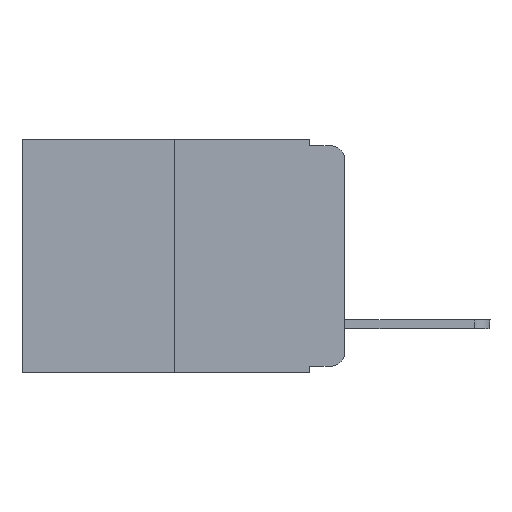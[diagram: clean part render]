
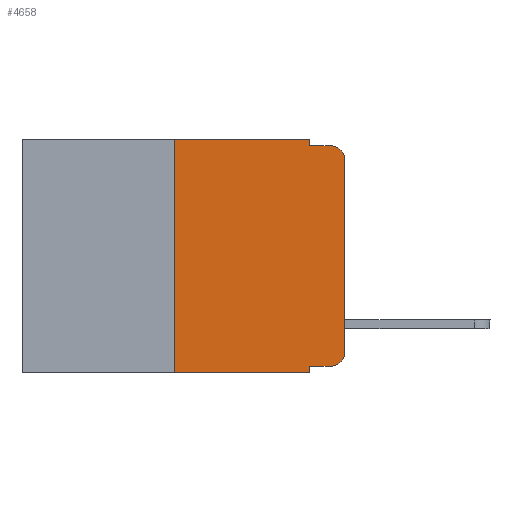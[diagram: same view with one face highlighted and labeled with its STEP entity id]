
A CAD part, left-side view. The second image highlights one B-rep face of the part: STEP entity #4658.
In plain terms, the highlighted planar face has unit normal (-1, 0, 0).
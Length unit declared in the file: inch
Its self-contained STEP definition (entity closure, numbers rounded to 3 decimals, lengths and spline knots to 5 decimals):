
#89 = VERTEX_POINT ( 'NONE', #10293 ) ;
#838 = PLANE ( 'NONE',  #9090 ) ;
#1021 = LINE ( 'NONE', #12332, #5460 ) ;
#1070 = DIRECTION ( 'NONE',  ( 0., 0., 1. ) ) ;
#1566 = VERTEX_POINT ( 'NONE', #2214 ) ;
#1743 = ORIENTED_EDGE ( 'NONE', *, *, #5074, .F. ) ;
#1755 = CARTESIAN_POINT ( 'NONE',  ( 0., 0.02, -0.333 ) ) ;
#2003 = AXIS2_PLACEMENT_3D ( 'NONE', #7945, #13956, #18308 ) ;
#2105 = VERTEX_POINT ( 'NONE', #3753 ) ;
#2194 = CIRCLE ( 'NONE', #2003, 0.02 ) ;
#2214 = CARTESIAN_POINT ( 'NONE',  ( 0., 0.051, -0.01 ) ) ;
#2468 = VECTOR ( 'NONE', #13361, 39.37008 ) ;
#2603 = EDGE_CURVE ( 'NONE', #1566, #3962, #10765, .T. ) ;
#2634 = EDGE_CURVE ( 'NONE', #2105, #3428, #10291, .T. ) ;
#3071 = CIRCLE ( 'NONE', #10545, 0.02 ) ;
#3290 = EDGE_CURVE ( 'NONE', #9376, #14216, #14406, .T. ) ;
#3428 = VERTEX_POINT ( 'NONE', #13125 ) ;
#3642 = EDGE_CURVE ( 'NONE', #2105, #6803, #9909, .T. ) ;
#3753 = CARTESIAN_POINT ( 'NONE',  ( 0., 0.25, -0.343 ) ) ;
#3795 = DIRECTION ( 'NONE',  ( 1., 0., 0. ) ) ;
#3962 = VERTEX_POINT ( 'NONE', #6539 ) ;
#4076 = DIRECTION ( 'NONE',  ( 0., -1., 0. ) ) ;
#4378 = DIRECTION ( 'NONE',  ( 0., 0., -1. ) ) ;
#4658 = ADVANCED_FACE ( 'NONE', ( #15399 ), #838, .F. ) ;
#5074 = EDGE_CURVE ( 'NONE', #16321, #1566, #13083, .T. ) ;
#5187 = CARTESIAN_POINT ( 'NONE',  ( 0., 0., -0.313 ) ) ;
#5460 = VECTOR ( 'NONE', #12212, 39.37008 ) ;
#5867 = ORIENTED_EDGE ( 'NONE', *, *, #18678, .F. ) ;
#5952 = EDGE_CURVE ( 'NONE', #89, #3428, #1021, .T. ) ;
#6423 = EDGE_CURVE ( 'NONE', #89, #9762, #7309, .T. ) ;
#6539 = CARTESIAN_POINT ( 'NONE',  ( 0., 0.02, -0.01 ) ) ;
#6640 = LINE ( 'NONE', #13337, #9137 ) ;
#6751 = VECTOR ( 'NONE', #10301, 39.37008 ) ;
#6803 = VERTEX_POINT ( 'NONE', #10557 ) ;
#7309 = LINE ( 'NONE', #12867, #12792 ) ;
#7557 = CARTESIAN_POINT ( 'NONE',  ( 0., 0., -0.03 ) ) ;
#7945 = CARTESIAN_POINT ( 'NONE',  ( 0., 0.02, -0.03 ) ) ;
#8601 = CARTESIAN_POINT ( 'NONE',  ( 0., 0., 0. ) ) ;
#9060 = DIRECTION ( 'NONE',  ( 0., -1., 0. ) ) ;
#9090 = AXIS2_PLACEMENT_3D ( 'NONE', #11155, #3795, #12777 ) ;
#9137 = VECTOR ( 'NONE', #11846, 39.37008 ) ;
#9376 = VERTEX_POINT ( 'NONE', #5187 ) ;
#9450 = EDGE_LOOP ( 'NONE', ( #17713, #18507, #15532, #1743, #5867, #17022, #13806, #9598, #11531, #18291 ) ) ;
#9598 = ORIENTED_EDGE ( 'NONE', *, *, #5952, .F. ) ;
#9762 = VERTEX_POINT ( 'NONE', #1755 ) ;
#9814 = DIRECTION ( 'NONE',  ( -1., 0., 0. ) ) ;
#9909 = LINE ( 'NONE', #19089, #6751 ) ;
#10291 = LINE ( 'NONE', #10540, #12130 ) ;
#10293 = CARTESIAN_POINT ( 'NONE',  ( 0., 0.051, -0.333 ) ) ;
#10301 = DIRECTION ( 'NONE',  ( 0., 0., 1. ) ) ;
#10540 = CARTESIAN_POINT ( 'NONE',  ( 0., 0.473, -0.343 ) ) ;
#10545 = AXIS2_PLACEMENT_3D ( 'NONE', #18872, #9814, #17382 ) ;
#10557 = CARTESIAN_POINT ( 'NONE',  ( 0., 0.25, 0. ) ) ;
#10765 = LINE ( 'NONE', #14967, #2468 ) ;
#11155 = CARTESIAN_POINT ( 'NONE',  ( 0., 0.473, 0. ) ) ;
#11531 = ORIENTED_EDGE ( 'NONE', *, *, #6423, .T. ) ;
#11613 = CARTESIAN_POINT ( 'NONE',  ( 0., 0.051, 0. ) ) ;
#11846 = DIRECTION ( 'NONE',  ( 0., -1., 0. ) ) ;
#12130 = VECTOR ( 'NONE', #9060, 39.37008 ) ;
#12212 = DIRECTION ( 'NONE',  ( 0., 0., -1. ) ) ;
#12332 = CARTESIAN_POINT ( 'NONE',  ( 0., 0.051, 0. ) ) ;
#12661 = EDGE_CURVE ( 'NONE', #14216, #3962, #2194, .T. ) ;
#12777 = DIRECTION ( 'NONE',  ( 0., 0., -1. ) ) ;
#12792 = VECTOR ( 'NONE', #4076, 39.37008 ) ;
#12843 = VECTOR ( 'NONE', #4378, 39.37008 ) ;
#12867 = CARTESIAN_POINT ( 'NONE',  ( 0., 0.051, -0.333 ) ) ;
#13083 = LINE ( 'NONE', #11613, #12843 ) ;
#13125 = CARTESIAN_POINT ( 'NONE',  ( 0., 0.051, -0.343 ) ) ;
#13337 = CARTESIAN_POINT ( 'NONE',  ( 0., 0.473, 0. ) ) ;
#13361 = DIRECTION ( 'NONE',  ( 0., -1., 0. ) ) ;
#13806 = ORIENTED_EDGE ( 'NONE', *, *, #2634, .T. ) ;
#13956 = DIRECTION ( 'NONE',  ( -1., 0., 0. ) ) ;
#14216 = VERTEX_POINT ( 'NONE', #7557 ) ;
#14374 = EDGE_CURVE ( 'NONE', #9762, #9376, #3071, .T. ) ;
#14406 = LINE ( 'NONE', #8601, #18884 ) ;
#14967 = CARTESIAN_POINT ( 'NONE',  ( 0., 0.051, -0.01 ) ) ;
#15399 = FACE_OUTER_BOUND ( 'NONE', #9450, .T. ) ;
#15492 = CARTESIAN_POINT ( 'NONE',  ( 0., 0.051, 0. ) ) ;
#15532 = ORIENTED_EDGE ( 'NONE', *, *, #2603, .F. ) ;
#16321 = VERTEX_POINT ( 'NONE', #15492 ) ;
#17022 = ORIENTED_EDGE ( 'NONE', *, *, #3642, .F. ) ;
#17382 = DIRECTION ( 'NONE',  ( 0., 0., -1. ) ) ;
#17713 = ORIENTED_EDGE ( 'NONE', *, *, #3290, .T. ) ;
#18291 = ORIENTED_EDGE ( 'NONE', *, *, #14374, .T. ) ;
#18308 = DIRECTION ( 'NONE',  ( 0., 0., -1. ) ) ;
#18507 = ORIENTED_EDGE ( 'NONE', *, *, #12661, .T. ) ;
#18678 = EDGE_CURVE ( 'NONE', #6803, #16321, #6640, .T. ) ;
#18872 = CARTESIAN_POINT ( 'NONE',  ( 0., 0.02, -0.313 ) ) ;
#18884 = VECTOR ( 'NONE', #1070, 39.37008 ) ;
#19089 = CARTESIAN_POINT ( 'NONE',  ( 0., 0.25, 0. ) ) ;
